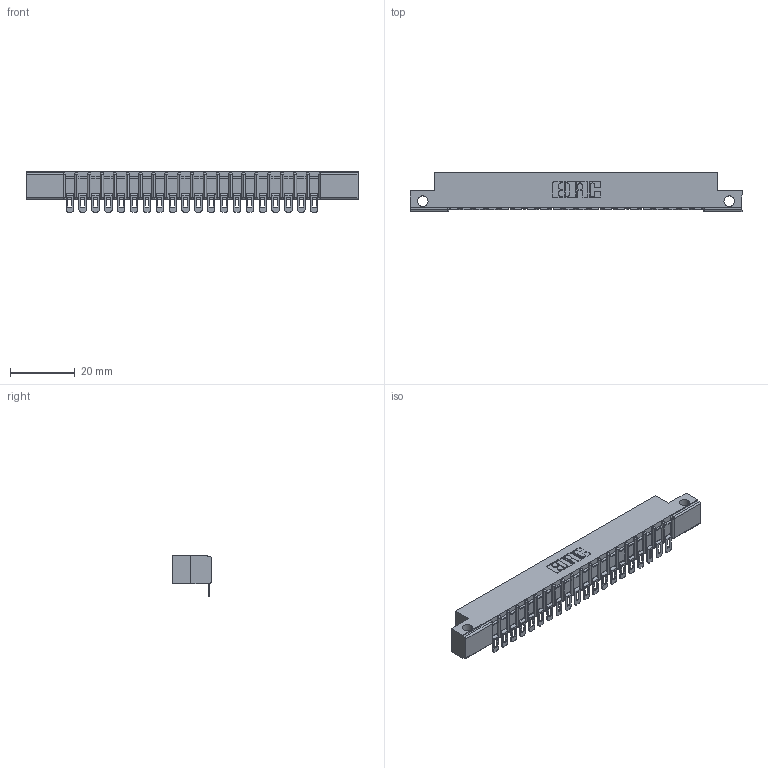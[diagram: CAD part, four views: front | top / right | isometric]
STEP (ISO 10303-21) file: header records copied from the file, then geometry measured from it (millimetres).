
FILE_DESCRIPTION (( 'STEP AP203' ), '1' );
FILE_NAME ('307-020-454-112.STEP', '2020-09-27T03:07:57', ( '' ), ( '' ), 'SwSTEP 2.0', 'SolidWorks 2020', '' );
FILE_SCHEMA (( 'CONFIG_CONTROL_DESIGN' ));
Length unit declared in the file: inch
Products named in the file (3): 307-290-002_554; 307-020-454-112; 307 Part_.128 Dia Side Mounting Holes
Assembly tree (21 placements, depth 2):
  307-020-454-112
    307 Part_.128 Dia Side Mounting Holes
    307-290-002_554  x20
Bounding box: 102.26 x 12.01 x 12.52 mm (x, y, z)
Volume: 6681.3 mm3; surface area: 11985.7 mm2
Topology: 21 solids, 21 shells, 1759 faces, 5383 edges, 3530 vertices
Faces by surface type: plane 990, cylinder 727, sphere 42
Entity records: 20825 total; most frequent: CARTESIAN_POINT 3510, ORIENTED_EDGE 3500, DIRECTION 3426, EDGE_CURVE 1750, LINE 1322, VECTOR 1322, VERTEX_POINT 1136, AXIS2_PLACEMENT_3D 1052
